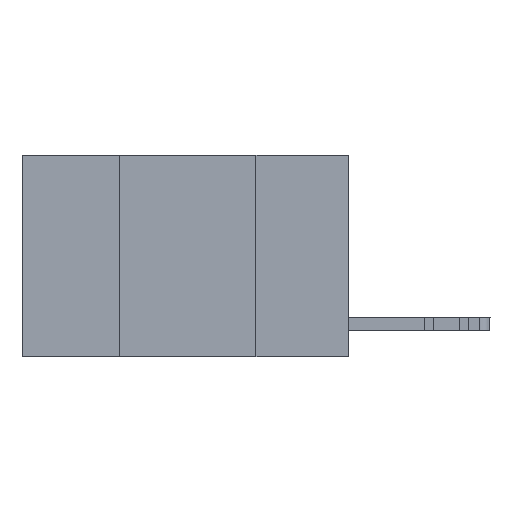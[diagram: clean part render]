
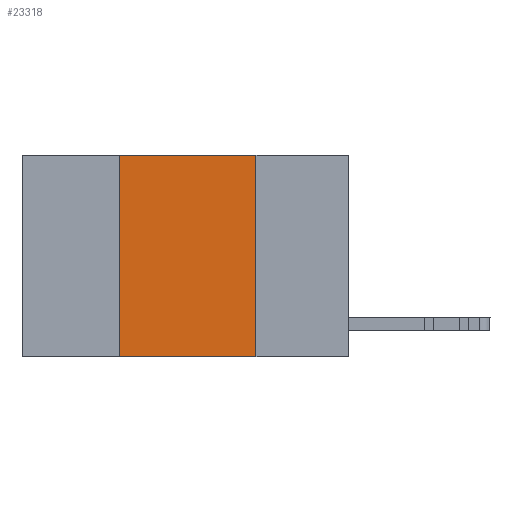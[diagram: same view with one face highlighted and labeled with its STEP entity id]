
A CAD part, left-side view. The second image highlights one B-rep face of the part: STEP entity #23318.
In plain terms, the highlighted planar face has unit normal (-1, 0, 0).
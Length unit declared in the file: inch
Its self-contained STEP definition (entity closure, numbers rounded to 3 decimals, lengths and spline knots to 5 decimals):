
#277 = VECTOR ( 'NONE', #28016, 39.37008 ) ;
#580 = CARTESIAN_POINT ( 'NONE',  ( 0., 0.6, -0.37 ) ) ;
#992 = LINE ( 'NONE', #580, #277 ) ;
#1458 = ORIENTED_EDGE ( 'NONE', *, *, #26757, .T. ) ;
#1575 = LINE ( 'NONE', #26744, #25200 ) ;
#1981 = EDGE_LOOP ( 'NONE', ( #24044, #5205, #28940, #1458 ) ) ;
#2620 = CARTESIAN_POINT ( 'NONE',  ( 0., 0.17, -0.37 ) ) ;
#3083 = VECTOR ( 'NONE', #26057, 39.37008 ) ;
#3715 = EDGE_CURVE ( 'NONE', #23036, #6579, #1575, .T. ) ;
#5205 = ORIENTED_EDGE ( 'NONE', *, *, #26598, .F. ) ;
#5348 = LINE ( 'NONE', #22967, #28129 ) ;
#6579 = VERTEX_POINT ( 'NONE', #24721 ) ;
#7812 = CARTESIAN_POINT ( 'NONE',  ( 0., 0.17, 0. ) ) ;
#8866 = EDGE_CURVE ( 'NONE', #10758, #13404, #9181, .T. ) ;
#9181 = LINE ( 'NONE', #7812, #3083 ) ;
#9742 = CARTESIAN_POINT ( 'NONE',  ( 0., 0.6, 0. ) ) ;
#9845 = PLANE ( 'NONE',  #21690 ) ;
#10758 = VERTEX_POINT ( 'NONE', #25048 ) ;
#12184 = DIRECTION ( 'NONE',  ( 0., 0., -1. ) ) ;
#12265 = FACE_OUTER_BOUND ( 'NONE', #1981, .T. ) ;
#13404 = VERTEX_POINT ( 'NONE', #2620 ) ;
#17779 = DIRECTION ( 'NONE',  ( 0., 0., 1. ) ) ;
#20388 = CARTESIAN_POINT ( 'NONE',  ( 0., 0.42, -0.37 ) ) ;
#21690 = AXIS2_PLACEMENT_3D ( 'NONE', #9742, #25829, #12184 ) ;
#22967 = CARTESIAN_POINT ( 'NONE',  ( 0., 0.6, 0. ) ) ;
#23036 = VERTEX_POINT ( 'NONE', #20388 ) ;
#23318 = ADVANCED_FACE ( 'NONE', ( #12265 ), #9845, .F. ) ;
#24044 = ORIENTED_EDGE ( 'NONE', *, *, #8866, .F. ) ;
#24721 = CARTESIAN_POINT ( 'NONE',  ( 0., 0.42, 0. ) ) ;
#25048 = CARTESIAN_POINT ( 'NONE',  ( 0., 0.17, 0. ) ) ;
#25200 = VECTOR ( 'NONE', #17779, 39.37008 ) ;
#25829 = DIRECTION ( 'NONE',  ( 1., 0., 0. ) ) ;
#26057 = DIRECTION ( 'NONE',  ( 0., 0., -1. ) ) ;
#26598 = EDGE_CURVE ( 'NONE', #6579, #10758, #5348, .T. ) ;
#26744 = CARTESIAN_POINT ( 'NONE',  ( 0., 0.42, 0. ) ) ;
#26757 = EDGE_CURVE ( 'NONE', #23036, #13404, #992, .T. ) ;
#27460 = DIRECTION ( 'NONE',  ( 0., -1., 0. ) ) ;
#28016 = DIRECTION ( 'NONE',  ( 0., -1., 0. ) ) ;
#28129 = VECTOR ( 'NONE', #27460, 39.37008 ) ;
#28940 = ORIENTED_EDGE ( 'NONE', *, *, #3715, .F. ) ;
